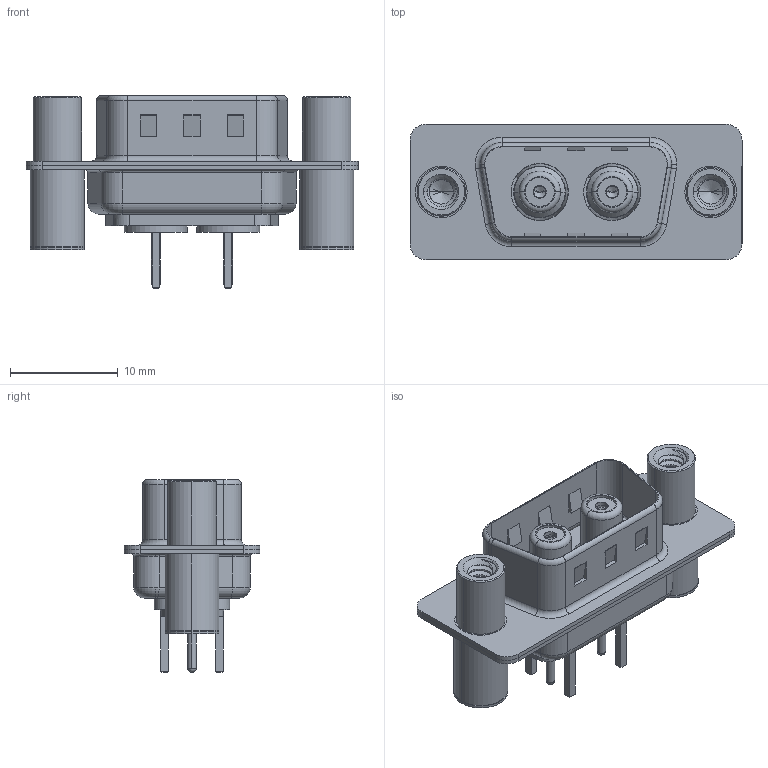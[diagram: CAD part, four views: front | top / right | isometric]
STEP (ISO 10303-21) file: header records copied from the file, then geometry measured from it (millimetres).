
FILE_DESCRIPTION (( 'STEP AP203' ), '1' );
FILE_NAME ('627-2W2-624-7N4.STEP', '2019-05-23T23:43:34', ( '' ), ( '' ), 'SwSTEP 2.0', 'SolidWorks 2016', '' );
FILE_SCHEMA (( 'CONFIG_CONTROL_DESIGN' ));
Length unit declared in the file: millimetre
Products named in the file (11): Locking Collar; Socket_Str; 627Combo Housing_2W2; Co-Ax Jack Assy_S; 627Combo Shell Rear_09 Contacts; 627-2W2-624-7N4; 627Combo Shell Front_09 Contacts; 627Combo Threaded Standoff and Board Spacer_4; Co-Ax Jack_Straight PC Tail; Insulator Socket; Insulator Socket 2
Assembly tree (12 placements, depth 3):
  627-2W2-624-7N4
    627Combo Housing_2W2
    627Combo Shell Rear_09 Contacts
    627Combo Shell Front_09 Contacts
    627Combo Threaded Standoff and Board Spacer_4  x2
    Co-Ax Jack Assy_S  x2
      Co-Ax Jack_Straight PC Tail
      Insulator Socket
      Insulator Socket 2
      Locking Collar
      Socket_Str
Bounding box: 30.8 x 12.6 x 17.9 mm (x, y, z)
Volume: 1644.6 mm3; surface area: 4930 mm2
Topology: 15 solids, 15 shells, 612 faces, 1481 edges, 924 vertices
Faces by surface type: cylinder 275, plane 207, torus 62, cone 48, bspline 16, sphere 4
Entity records: 15930 total; most frequent: CARTESIAN_POINT 4538, DIRECTION 2223, ORIENTED_EDGE 2080, EDGE_CURVE 1040, AXIS2_PLACEMENT_3D 857, VERTEX_POINT 655, LINE 509, VECTOR 509
